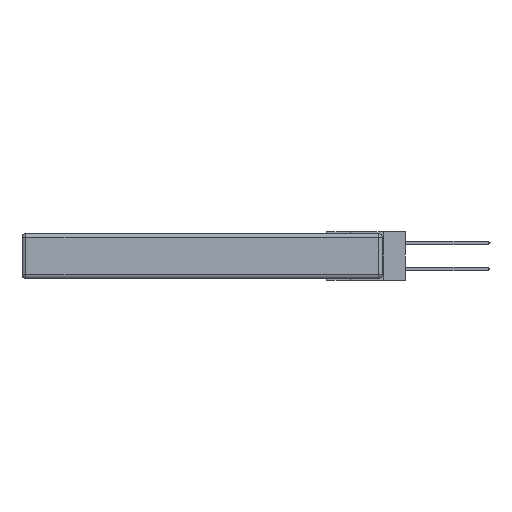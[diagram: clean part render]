
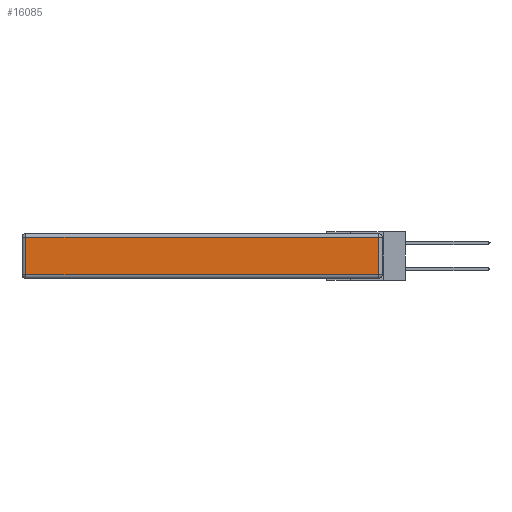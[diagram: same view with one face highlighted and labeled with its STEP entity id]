
A CAD part, left-side view. The second image highlights one B-rep face of the part: STEP entity #16085.
In plain terms, the highlighted planar face has unit normal (-1, 0, 0).
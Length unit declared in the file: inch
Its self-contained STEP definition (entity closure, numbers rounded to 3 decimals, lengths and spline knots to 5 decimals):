
#110 = CARTESIAN_POINT ( 'NONE',  ( 0., 2.72, -0.313 ) ) ;
#199 = VERTEX_POINT ( 'NONE', #24706 ) ;
#2066 = CARTESIAN_POINT ( 'NONE',  ( 0., 0.03, -0.313 ) ) ;
#2700 = VECTOR ( 'NONE', #19648, 39.37008 ) ;
#2958 = DIRECTION ( 'NONE',  ( 0., 0., 1. ) ) ;
#3532 = ORIENTED_EDGE ( 'NONE', *, *, #23258, .T. ) ;
#3667 = VECTOR ( 'NONE', #12054, 39.37008 ) ;
#4519 = VERTEX_POINT ( 'NONE', #110 ) ;
#7217 = CARTESIAN_POINT ( 'NONE',  ( 0., 2.75, -0.03 ) ) ;
#7739 = CARTESIAN_POINT ( 'NONE',  ( 0., 2.72, -0.343 ) ) ;
#8012 = LINE ( 'NONE', #7739, #2700 ) ;
#9615 = EDGE_CURVE ( 'NONE', #12824, #4519, #8012, .T. ) ;
#10227 = EDGE_CURVE ( 'NONE', #199, #12824, #15191, .T. ) ;
#11881 = DIRECTION ( 'NONE',  ( 0., 0., 1. ) ) ;
#12051 = VECTOR ( 'NONE', #13017, 39.37008 ) ;
#12054 = DIRECTION ( 'NONE',  ( 0., -1., 0. ) ) ;
#12729 = CARTESIAN_POINT ( 'NONE',  ( 0., 2.72, -0.03 ) ) ;
#12824 = VERTEX_POINT ( 'NONE', #12729 ) ;
#12920 = DIRECTION ( 'NONE',  ( -1., 0., 0. ) ) ;
#12997 = EDGE_LOOP ( 'NONE', ( #3532, #22888, #22952, #18547 ) ) ;
#13017 = DIRECTION ( 'NONE',  ( 0., 1., 0. ) ) ;
#13963 = CARTESIAN_POINT ( 'NONE',  ( 0., 0., -0.313 ) ) ;
#15191 = LINE ( 'NONE', #7217, #12051 ) ;
#15335 = VECTOR ( 'NONE', #11881, 39.37008 ) ;
#15491 = AXIS2_PLACEMENT_3D ( 'NONE', #22686, #12920, #2958 ) ;
#16085 = ADVANCED_FACE ( 'NONE', ( #19623 ), #18703, .T. ) ;
#18547 = ORIENTED_EDGE ( 'NONE', *, *, #9615, .T. ) ;
#18703 = PLANE ( 'NONE',  #15491 ) ;
#19623 = FACE_OUTER_BOUND ( 'NONE', #12997, .T. ) ;
#19648 = DIRECTION ( 'NONE',  ( 0., 0., -1. ) ) ;
#19703 = LINE ( 'NONE', #23590, #15335 ) ;
#20106 = EDGE_CURVE ( 'NONE', #21466, #199, #19703, .T. ) ;
#21466 = VERTEX_POINT ( 'NONE', #2066 ) ;
#22686 = CARTESIAN_POINT ( 'NONE',  ( 0., 0., -0.343 ) ) ;
#22888 = ORIENTED_EDGE ( 'NONE', *, *, #20106, .T. ) ;
#22952 = ORIENTED_EDGE ( 'NONE', *, *, #10227, .T. ) ;
#23258 = EDGE_CURVE ( 'NONE', #4519, #21466, #25785, .T. ) ;
#23590 = CARTESIAN_POINT ( 'NONE',  ( 0., 0.03, -0.343 ) ) ;
#24706 = CARTESIAN_POINT ( 'NONE',  ( 0., 0.03, -0.03 ) ) ;
#25785 = LINE ( 'NONE', #13963, #3667 ) ;
